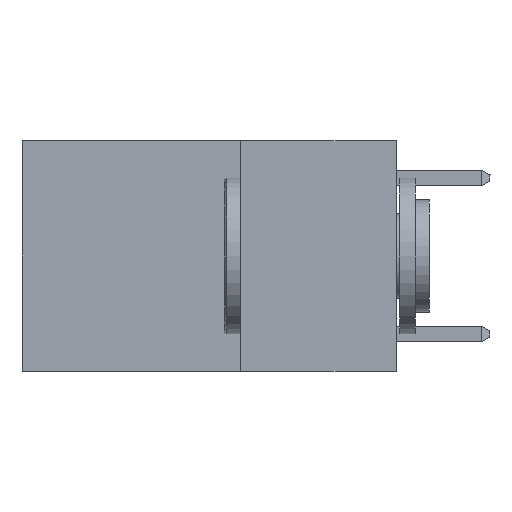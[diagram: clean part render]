
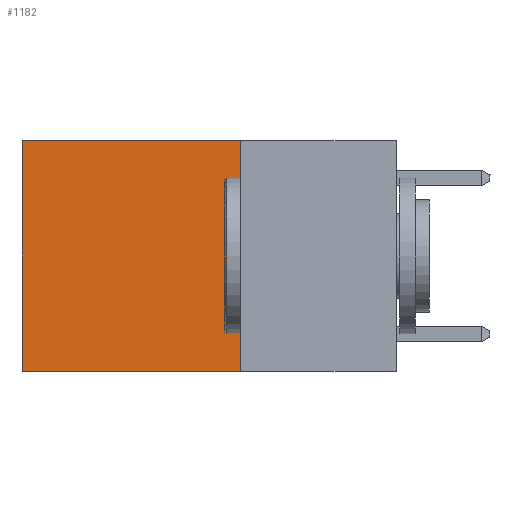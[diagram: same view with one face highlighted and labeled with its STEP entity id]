
A CAD part, left-side view. The second image highlights one B-rep face of the part: STEP entity #1182.
In plain terms, the highlighted planar face has unit normal (-1, 0, 0).
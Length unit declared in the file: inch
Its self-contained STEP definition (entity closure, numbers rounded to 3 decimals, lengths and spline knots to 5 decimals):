
#214 = ORIENTED_EDGE ( 'NONE', *, *, #9907, .T. ) ;
#218 = EDGE_LOOP ( 'NONE', ( #7327, #7587, #9897, #214 ) ) ;
#834 = LINE ( 'NONE', #3491, #3623 ) ;
#1168 = DIRECTION ( 'NONE',  ( 1., 0., 0. ) ) ;
#1182 = ADVANCED_FACE ( 'NONE', ( #7825 ), #5503, .F. ) ;
#1200 = EDGE_CURVE ( 'NONE', #2357, #3353, #2893, .T. ) ;
#1736 = AXIS2_PLACEMENT_3D ( 'NONE', #5208, #1168, #8912 ) ;
#2145 = VECTOR ( 'NONE', #8681, 39.37008 ) ;
#2357 = VERTEX_POINT ( 'NONE', #3425 ) ;
#2893 = LINE ( 'NONE', #10827, #5197 ) ;
#3353 = VERTEX_POINT ( 'NONE', #9629 ) ;
#3425 = CARTESIAN_POINT ( 'NONE',  ( 0.2625, 0.25, 0. ) ) ;
#3491 = CARTESIAN_POINT ( 'NONE',  ( 0.2625, 0.25, -0.37 ) ) ;
#3623 = VECTOR ( 'NONE', #9586, 39.37008 ) ;
#3898 = VECTOR ( 'NONE', #11188, 39.37008 ) ;
#4125 = EDGE_CURVE ( 'NONE', #9814, #9989, #10581, .T. ) ;
#5197 = VECTOR ( 'NONE', #8290, 39.37008 ) ;
#5208 = CARTESIAN_POINT ( 'NONE',  ( 0.2625, 0.25, 0. ) ) ;
#5503 = PLANE ( 'NONE',  #1736 ) ;
#6966 = CARTESIAN_POINT ( 'NONE',  ( 0.2625, 0.6, 0. ) ) ;
#7327 = ORIENTED_EDGE ( 'NONE', *, *, #4125, .T. ) ;
#7587 = ORIENTED_EDGE ( 'NONE', *, *, #9960, .F. ) ;
#7825 = FACE_OUTER_BOUND ( 'NONE', #218, .T. ) ;
#8290 = DIRECTION ( 'NONE',  ( 0., 0., -1. ) ) ;
#8556 = LINE ( 'NONE', #10346, #3898 ) ;
#8681 = DIRECTION ( 'NONE',  ( 0., 0., -1. ) ) ;
#8912 = DIRECTION ( 'NONE',  ( 0., 0., -1. ) ) ;
#9586 = DIRECTION ( 'NONE',  ( 0., 1., 0. ) ) ;
#9625 = CARTESIAN_POINT ( 'NONE',  ( 0.2625, 0.6, -0.37 ) ) ;
#9629 = CARTESIAN_POINT ( 'NONE',  ( 0.2625, 0.25, -0.37 ) ) ;
#9814 = VERTEX_POINT ( 'NONE', #11035 ) ;
#9897 = ORIENTED_EDGE ( 'NONE', *, *, #1200, .F. ) ;
#9907 = EDGE_CURVE ( 'NONE', #2357, #9814, #8556, .T. ) ;
#9960 = EDGE_CURVE ( 'NONE', #3353, #9989, #834, .T. ) ;
#9989 = VERTEX_POINT ( 'NONE', #9625 ) ;
#10346 = CARTESIAN_POINT ( 'NONE',  ( 0.2625, 0.25, 0. ) ) ;
#10581 = LINE ( 'NONE', #6966, #2145 ) ;
#10827 = CARTESIAN_POINT ( 'NONE',  ( 0.2625, 0.25, 0. ) ) ;
#11035 = CARTESIAN_POINT ( 'NONE',  ( 0.2625, 0.6, 0. ) ) ;
#11188 = DIRECTION ( 'NONE',  ( 0., 1., 0. ) ) ;
